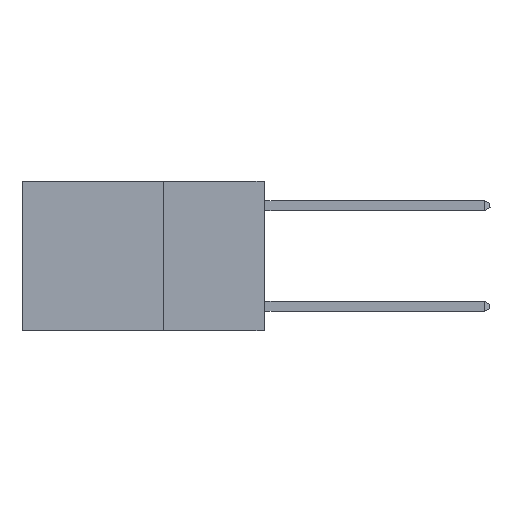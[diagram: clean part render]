
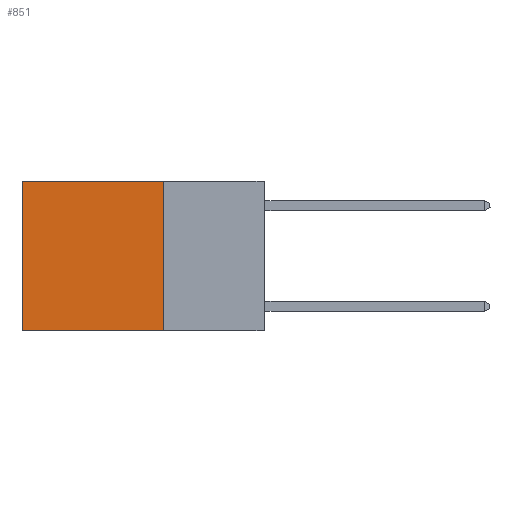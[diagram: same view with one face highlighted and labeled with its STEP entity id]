
A CAD part, left-side view. The second image highlights one B-rep face of the part: STEP entity #851.
In plain terms, the highlighted planar face has unit normal (-1, 0, 0).
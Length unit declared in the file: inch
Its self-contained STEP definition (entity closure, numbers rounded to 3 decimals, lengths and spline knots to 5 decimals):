
#126 = ORIENTED_EDGE ( 'NONE', *, *, #767, .T. ) ;
#564 = VECTOR ( 'NONE', #7698, 39.37008 ) ;
#746 = FACE_OUTER_BOUND ( 'NONE', #10519, .T. ) ;
#767 = EDGE_CURVE ( 'NONE', #5782, #5647, #11640, .T. ) ;
#831 = EDGE_CURVE ( 'NONE', #5782, #1819, #2145, .T. ) ;
#851 = ADVANCED_FACE ( 'NONE', ( #746 ), #5276, .F. ) ;
#1116 = CARTESIAN_POINT ( 'NONE',  ( 0.2625, 0.25, 0. ) ) ;
#1158 = DIRECTION ( 'NONE',  ( 0., 0., -1. ) ) ;
#1675 = CARTESIAN_POINT ( 'NONE',  ( 0.2625, 0.25, -0.37 ) ) ;
#1819 = VERTEX_POINT ( 'NONE', #4812 ) ;
#2011 = LINE ( 'NONE', #10106, #7250 ) ;
#2145 = LINE ( 'NONE', #11532, #7061 ) ;
#4812 = CARTESIAN_POINT ( 'NONE',  ( 0.2625, 0.25, -0.37 ) ) ;
#5276 = PLANE ( 'NONE',  #5895 ) ;
#5629 = ORIENTED_EDGE ( 'NONE', *, *, #6431, .T. ) ;
#5647 = VERTEX_POINT ( 'NONE', #8748 ) ;
#5782 = VERTEX_POINT ( 'NONE', #1116 ) ;
#5895 = AXIS2_PLACEMENT_3D ( 'NONE', #7334, #8393, #1158 ) ;
#5931 = DIRECTION ( 'NONE',  ( 0., 0., -1. ) ) ;
#6431 = EDGE_CURVE ( 'NONE', #5647, #7432, #2011, .T. ) ;
#7061 = VECTOR ( 'NONE', #10506, 39.37008 ) ;
#7139 = EDGE_CURVE ( 'NONE', #1819, #7432, #8314, .T. ) ;
#7153 = CARTESIAN_POINT ( 'NONE',  ( 0.2625, 0.25, 0. ) ) ;
#7250 = VECTOR ( 'NONE', #5931, 39.37008 ) ;
#7334 = CARTESIAN_POINT ( 'NONE',  ( 0.2625, 0.25, 0. ) ) ;
#7432 = VERTEX_POINT ( 'NONE', #10269 ) ;
#7698 = DIRECTION ( 'NONE',  ( 0., 1., 0. ) ) ;
#8314 = LINE ( 'NONE', #1675, #13196 ) ;
#8393 = DIRECTION ( 'NONE',  ( 1., 0., 0. ) ) ;
#8748 = CARTESIAN_POINT ( 'NONE',  ( 0.2625, 0.6, 0. ) ) ;
#9132 = DIRECTION ( 'NONE',  ( 0., 1., 0. ) ) ;
#9275 = ORIENTED_EDGE ( 'NONE', *, *, #7139, .F. ) ;
#10106 = CARTESIAN_POINT ( 'NONE',  ( 0.2625, 0.6, 0. ) ) ;
#10269 = CARTESIAN_POINT ( 'NONE',  ( 0.2625, 0.6, -0.37 ) ) ;
#10506 = DIRECTION ( 'NONE',  ( 0., 0., -1. ) ) ;
#10519 = EDGE_LOOP ( 'NONE', ( #5629, #9275, #11937, #126 ) ) ;
#11532 = CARTESIAN_POINT ( 'NONE',  ( 0.2625, 0.25, 0. ) ) ;
#11640 = LINE ( 'NONE', #7153, #564 ) ;
#11937 = ORIENTED_EDGE ( 'NONE', *, *, #831, .F. ) ;
#13196 = VECTOR ( 'NONE', #9132, 39.37008 ) ;
